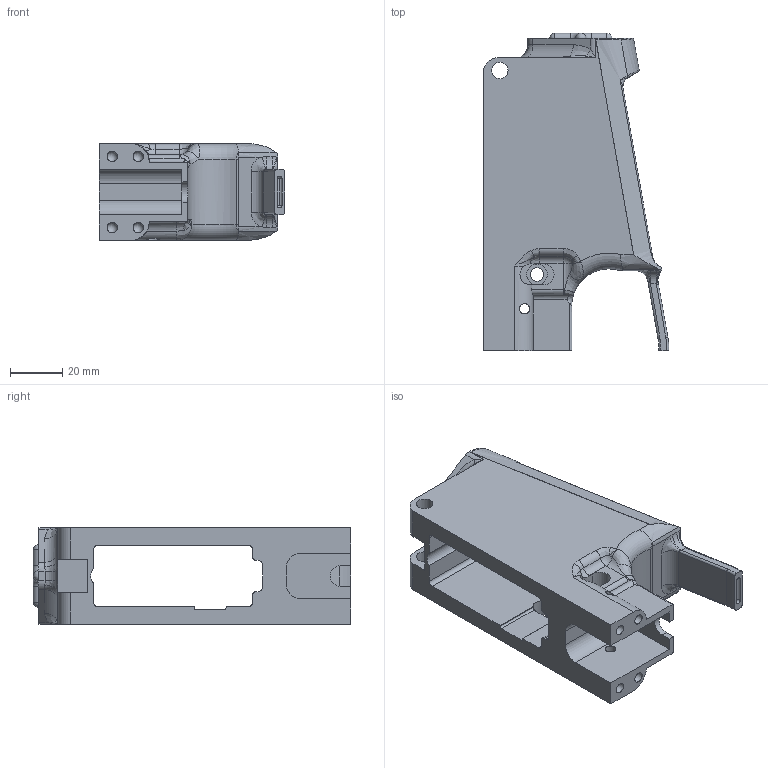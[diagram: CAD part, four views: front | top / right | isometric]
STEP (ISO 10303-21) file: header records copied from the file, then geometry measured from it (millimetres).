
FILE_DESCRIPTION (( 'STEP AP214' ), '1' );
FILE_NAME ('Atlas_DMR_Receiver_Front_V2.step', '2016-01-25T18:16:58', ( 'WarFairy' ), ( '' ), 'SwSTEP 2.0', 'SolidWorks 2015', '' );
FILE_SCHEMA (( 'AUTOMOTIVE_DESIGN' ));
Length unit declared in the file: millimetre
Products named in the file (1): Atlas_DMR_Receiver_Front_V2
Bounding box: 71.28 x 122.01 x 37.13 mm (x, y, z)
Volume: 111277.2 mm3; surface area: 36068.3 mm2
Topology: 1 solids, 1 shells, 238 faces, 647 edges, 392 vertices
Faces by surface type: cylinder 80, plane 69, bspline 64, torus 15, sphere 10
Full cylindrical faces by diameter (mm): 3.969 x2, 5.182 x1, 6.375 x2, 7.938 x1
Entity records: 9928 total; most frequent: CARTESIAN_POINT 4554, ORIENTED_EDGE 1220, DIRECTION 981, EDGE_CURVE 610, VERTEX_POINT 384, AXIS2_PLACEMENT_3D 357, LINE 267, VECTOR 267
